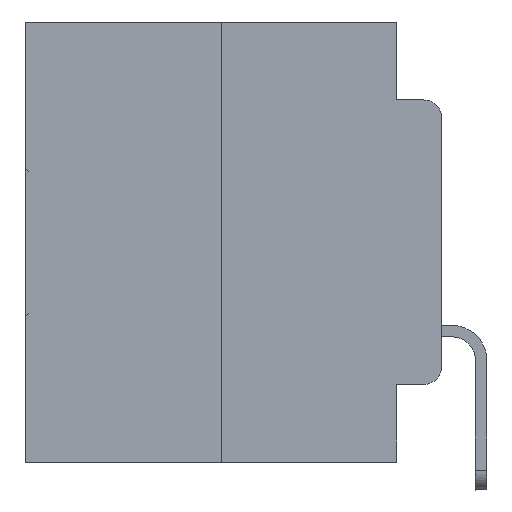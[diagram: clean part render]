
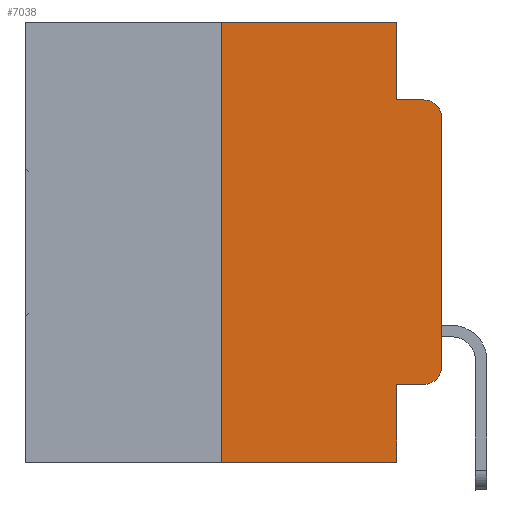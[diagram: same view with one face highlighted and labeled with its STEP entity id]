
A CAD part, left-side view. The second image highlights one B-rep face of the part: STEP entity #7038.
In plain terms, the highlighted planar face has unit normal (-1, 0, 0).
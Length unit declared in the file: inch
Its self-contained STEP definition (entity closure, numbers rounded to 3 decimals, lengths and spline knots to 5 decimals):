
#415 = ORIENTED_EDGE ( 'NONE', *, *, #12484, .F. ) ;
#996 = EDGE_CURVE ( 'NONE', #29155, #8152, #13212, .T. ) ;
#1078 = DIRECTION ( 'NONE',  ( -1., 0., 0. ) ) ;
#1339 = LINE ( 'NONE', #27627, #12592 ) ;
#2201 = PLANE ( 'NONE',  #28618 ) ;
#3222 = DIRECTION ( 'NONE',  ( 0., -1., 0. ) ) ;
#3501 = ORIENTED_EDGE ( 'NONE', *, *, #14711, .F. ) ;
#3608 = CARTESIAN_POINT ( 'NONE',  ( 0., 0.02, -0.0885 ) ) ;
#3695 = VECTOR ( 'NONE', #11536, 39.37008 ) ;
#4095 = LINE ( 'NONE', #29331, #12454 ) ;
#4193 = CARTESIAN_POINT ( 'NONE',  ( 0., 0., 0. ) ) ;
#4218 = EDGE_CURVE ( 'NONE', #8152, #28533, #10654, .T. ) ;
#4253 = DIRECTION ( 'NONE',  ( 0., 0., -1. ) ) ;
#4428 = EDGE_CURVE ( 'NONE', #16066, #17900, #14274, .T. ) ;
#5268 = CARTESIAN_POINT ( 'NONE',  ( 0., 0.051, -0.4115 ) ) ;
#5400 = VERTEX_POINT ( 'NONE', #5268 ) ;
#5756 = CARTESIAN_POINT ( 'NONE',  ( 0., 0.051, -0.5 ) ) ;
#6359 = LINE ( 'NONE', #15700, #25979 ) ;
#7038 = ADVANCED_FACE ( 'NONE', ( #28030 ), #2201, .F. ) ;
#7303 = CARTESIAN_POINT ( 'NONE',  ( 0., 0.02, -0.4115 ) ) ;
#8152 = VERTEX_POINT ( 'NONE', #20007 ) ;
#8600 = CARTESIAN_POINT ( 'NONE',  ( 0., 0.25, -0.5 ) ) ;
#8650 = ORIENTED_EDGE ( 'NONE', *, *, #28090, .T. ) ;
#9460 = ORIENTED_EDGE ( 'NONE', *, *, #4218, .T. ) ;
#9611 = AXIS2_PLACEMENT_3D ( 'NONE', #19108, #12082, #28974 ) ;
#9620 = EDGE_CURVE ( 'NONE', #17900, #23014, #11696, .T. ) ;
#10277 = AXIS2_PLACEMENT_3D ( 'NONE', #22050, #1078, #17159 ) ;
#10393 = VECTOR ( 'NONE', #20861, 39.37008 ) ;
#10538 = VECTOR ( 'NONE', #12700, 39.37008 ) ;
#10654 = LINE ( 'NONE', #4193, #22165 ) ;
#11536 = DIRECTION ( 'NONE',  ( 0., 0., 1. ) ) ;
#11547 = CARTESIAN_POINT ( 'NONE',  ( 0., 0.473, 0. ) ) ;
#11548 = DIRECTION ( 'NONE',  ( 0., 0., -1. ) ) ;
#11696 = LINE ( 'NONE', #11547, #10393 ) ;
#11722 = EDGE_CURVE ( 'NONE', #28533, #23418, #26171, .T. ) ;
#12082 = DIRECTION ( 'NONE',  ( -1., 0., 0. ) ) ;
#12454 = VECTOR ( 'NONE', #20454, 39.37008 ) ;
#12484 = EDGE_CURVE ( 'NONE', #13129, #23418, #24449, .T. ) ;
#12592 = VECTOR ( 'NONE', #4253, 39.37008 ) ;
#12700 = DIRECTION ( 'NONE',  ( 0., -1., 0. ) ) ;
#13129 = VERTEX_POINT ( 'NONE', #26444 ) ;
#13212 = CIRCLE ( 'NONE', #10277, 0.02 ) ;
#14274 = LINE ( 'NONE', #27875, #3695 ) ;
#14711 = EDGE_CURVE ( 'NONE', #23014, #13129, #1339, .T. ) ;
#14854 = CARTESIAN_POINT ( 'NONE',  ( 0., 0.051, 0. ) ) ;
#14974 = CARTESIAN_POINT ( 'NONE',  ( 0., 0.051, -0.0885 ) ) ;
#14998 = VERTEX_POINT ( 'NONE', #5756 ) ;
#15150 = CARTESIAN_POINT ( 'NONE',  ( 0., 0.051, -0.4115 ) ) ;
#15339 = CARTESIAN_POINT ( 'NONE',  ( 0., 0., -0.1085 ) ) ;
#15700 = CARTESIAN_POINT ( 'NONE',  ( 0., 0.473, -0.5 ) ) ;
#15712 = ORIENTED_EDGE ( 'NONE', *, *, #11722, .T. ) ;
#16066 = VERTEX_POINT ( 'NONE', #8600 ) ;
#16141 = CARTESIAN_POINT ( 'NONE',  ( 0., 0.473, 0. ) ) ;
#17159 = DIRECTION ( 'NONE',  ( 0., 0., -1. ) ) ;
#17900 = VERTEX_POINT ( 'NONE', #28303 ) ;
#17984 = ORIENTED_EDGE ( 'NONE', *, *, #4428, .F. ) ;
#19108 = CARTESIAN_POINT ( 'NONE',  ( 0., 0.02, -0.1085 ) ) ;
#19801 = DIRECTION ( 'NONE',  ( 0., 0., 1. ) ) ;
#20007 = CARTESIAN_POINT ( 'NONE',  ( 0., 0., -0.3915 ) ) ;
#20454 = DIRECTION ( 'NONE',  ( 0., 0., -1. ) ) ;
#20861 = DIRECTION ( 'NONE',  ( 0., -1., 0. ) ) ;
#21034 = EDGE_CURVE ( 'NONE', #16066, #14998, #6359, .T. ) ;
#21170 = DIRECTION ( 'NONE',  ( 1., 0., 0. ) ) ;
#21500 = ORIENTED_EDGE ( 'NONE', *, *, #9620, .F. ) ;
#22050 = CARTESIAN_POINT ( 'NONE',  ( 0., 0.02, -0.3915 ) ) ;
#22165 = VECTOR ( 'NONE', #19801, 39.37008 ) ;
#23011 = ORIENTED_EDGE ( 'NONE', *, *, #996, .T. ) ;
#23014 = VERTEX_POINT ( 'NONE', #14854 ) ;
#23247 = VECTOR ( 'NONE', #24468, 39.37008 ) ;
#23418 = VERTEX_POINT ( 'NONE', #3608 ) ;
#24449 = LINE ( 'NONE', #14974, #10538 ) ;
#24468 = DIRECTION ( 'NONE',  ( 0., -1., 0. ) ) ;
#25739 = ORIENTED_EDGE ( 'NONE', *, *, #21034, .T. ) ;
#25979 = VECTOR ( 'NONE', #3222, 39.37008 ) ;
#26171 = CIRCLE ( 'NONE', #9611, 0.02 ) ;
#26444 = CARTESIAN_POINT ( 'NONE',  ( 0., 0.051, -0.0885 ) ) ;
#26759 = LINE ( 'NONE', #15150, #23247 ) ;
#27368 = EDGE_CURVE ( 'NONE', #5400, #14998, #4095, .T. ) ;
#27627 = CARTESIAN_POINT ( 'NONE',  ( 0., 0.051, 0. ) ) ;
#27875 = CARTESIAN_POINT ( 'NONE',  ( 0., 0.25, 0. ) ) ;
#28030 = FACE_OUTER_BOUND ( 'NONE', #30038, .T. ) ;
#28090 = EDGE_CURVE ( 'NONE', #5400, #29155, #26759, .T. ) ;
#28303 = CARTESIAN_POINT ( 'NONE',  ( 0., 0.25, 0. ) ) ;
#28533 = VERTEX_POINT ( 'NONE', #15339 ) ;
#28618 = AXIS2_PLACEMENT_3D ( 'NONE', #16141, #21170, #11548 ) ;
#28974 = DIRECTION ( 'NONE',  ( 0., 0., -1. ) ) ;
#29155 = VERTEX_POINT ( 'NONE', #7303 ) ;
#29331 = CARTESIAN_POINT ( 'NONE',  ( 0., 0.051, 0. ) ) ;
#29479 = ORIENTED_EDGE ( 'NONE', *, *, #27368, .F. ) ;
#30038 = EDGE_LOOP ( 'NONE', ( #9460, #15712, #415, #3501, #21500, #17984, #25739, #29479, #8650, #23011 ) ) ;
